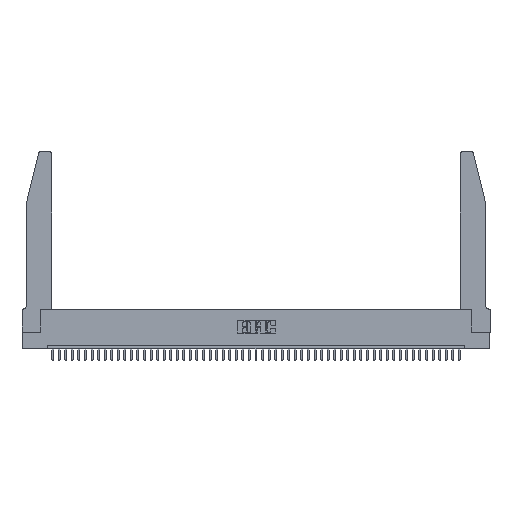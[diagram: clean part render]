
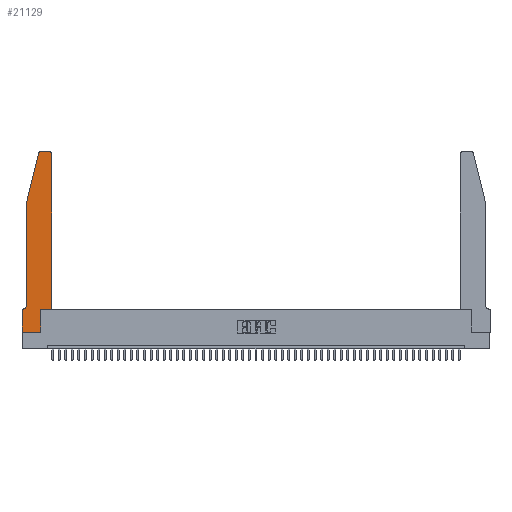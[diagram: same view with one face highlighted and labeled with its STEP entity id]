
A CAD part, top view. The second image highlights one B-rep face of the part: STEP entity #21129.
In plain terms, the highlighted planar face has unit normal (0, 0, 1).
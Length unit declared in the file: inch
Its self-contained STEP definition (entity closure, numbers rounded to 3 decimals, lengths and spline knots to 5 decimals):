
#786 = ORIENTED_EDGE ( 'NONE', *, *, #8176, .T. ) ;
#2566 = DIRECTION ( 'NONE',  ( 1., 0., 0. ) ) ;
#2634 = EDGE_CURVE ( 'NONE', #43806, #20962, #25922, .T. ) ;
#2810 = DIRECTION ( 'NONE',  ( 0., -1., 0. ) ) ;
#3086 = DIRECTION ( 'NONE',  ( 1., 0., 0. ) ) ;
#3744 = VECTOR ( 'NONE', #28747, 39.37008 ) ;
#3785 = CARTESIAN_POINT ( 'NONE',  ( 0.2865, 0.35, 0.37 ) ) ;
#3794 = VERTEX_POINT ( 'NONE', #37630 ) ;
#4685 = EDGE_CURVE ( 'NONE', #48485, #11136, #18845, .T. ) ;
#4690 = EDGE_CURVE ( 'NONE', #10500, #24135, #42140, .T. ) ;
#5651 = EDGE_CURVE ( 'NONE', #22814, #15166, #36626, .T. ) ;
#6064 = CIRCLE ( 'NONE', #27323, 0.03 ) ;
#6842 = DIRECTION ( 'NONE',  ( -1., 0., 0. ) ) ;
#6861 = CARTESIAN_POINT ( 'NONE',  ( 0.0055, 0.35, 0.37 ) ) ;
#7062 = CARTESIAN_POINT ( 'NONE',  ( 0.284, 2.72, 0.37 ) ) ;
#7360 = DIRECTION ( 'NONE',  ( 0., 1., 0. ) ) ;
#7755 = CARTESIAN_POINT ( 'NONE',  ( 0.4505, 0.35, 0.37 ) ) ;
#8176 = EDGE_CURVE ( 'NONE', #20939, #10500, #29077, .T. ) ;
#8830 = VECTOR ( 'NONE', #18913, 39.37008 ) ;
#8953 = CARTESIAN_POINT ( 'NONE',  ( 0., 0.35, 0.37 ) ) ;
#9318 = ORIENTED_EDGE ( 'NONE', *, *, #38672, .T. ) ;
#9411 = ORIENTED_EDGE ( 'NONE', *, *, #49438, .T. ) ;
#10112 = VECTOR ( 'NONE', #2810, 39.37008 ) ;
#10374 = AXIS2_PLACEMENT_3D ( 'NONE', #46440, #11872, #15708 ) ;
#10500 = VERTEX_POINT ( 'NONE', #46540 ) ;
#10507 = VECTOR ( 'NONE', #21748, 39.37008 ) ;
#10679 = CARTESIAN_POINT ( 'NONE',  ( 0., 0.35, 0.37 ) ) ;
#11030 = CIRCLE ( 'NONE', #30099, 0.03 ) ;
#11136 = VERTEX_POINT ( 'NONE', #22703 ) ;
#11353 = ORIENTED_EDGE ( 'NONE', *, *, #36166, .T. ) ;
#11358 = LINE ( 'NONE', #40221, #37043 ) ;
#11459 = DIRECTION ( 'NONE',  ( -1., 0., 0. ) ) ;
#11872 = DIRECTION ( 'NONE',  ( 0., 0., -1. ) ) ;
#12272 = CARTESIAN_POINT ( 'NONE',  ( 0.0755, 2., 0.37 ) ) ;
#12304 = LINE ( 'NONE', #49321, #35554 ) ;
#13378 = EDGE_CURVE ( 'NONE', #24135, #41936, #22000, .T. ) ;
#13555 = ORIENTED_EDGE ( 'NONE', *, *, #2634, .T. ) ;
#13577 = VECTOR ( 'NONE', #11459, 39.37008 ) ;
#14092 = EDGE_CURVE ( 'NONE', #11136, #22814, #12304, .T. ) ;
#14748 = CARTESIAN_POINT ( 'NONE',  ( 0.4505, 0.35, 0.37 ) ) ;
#15166 = VERTEX_POINT ( 'NONE', #7755 ) ;
#15403 = EDGE_LOOP ( 'NONE', ( #13555, #43340, #9318, #786, #43519, #43462, #38502, #45732, #43210, #43714, #9411, #11353 ) ) ;
#15708 = DIRECTION ( 'NONE',  ( -1., 0., 0. ) ) ;
#15936 = CARTESIAN_POINT ( 'NONE',  ( 0., 0., 0.37 ) ) ;
#17171 = DIRECTION ( 'NONE',  ( -0.239, -0.971, 0. ) ) ;
#17868 = VECTOR ( 'NONE', #6842, 39.37008 ) ;
#18358 = DIRECTION ( 'NONE',  ( 0., 0., 1. ) ) ;
#18657 = FACE_OUTER_BOUND ( 'NONE', #15403, .T. ) ;
#18824 = DIRECTION ( 'NONE',  ( 0., 0., 1. ) ) ;
#18845 = LINE ( 'NONE', #45037, #27773 ) ;
#18913 = DIRECTION ( 'NONE',  ( 0., 1., 0. ) ) ;
#19234 = DIRECTION ( 'NONE',  ( 1., 0., 0. ) ) ;
#19627 = LINE ( 'NONE', #34392, #10112 ) ;
#20939 = VERTEX_POINT ( 'NONE', #12272 ) ;
#20962 = VERTEX_POINT ( 'NONE', #44047 ) ;
#21129 = ADVANCED_FACE ( 'NONE', ( #18657 ), #37215, .T. ) ;
#21478 = LINE ( 'NONE', #14748, #8830 ) ;
#21748 = DIRECTION ( 'NONE',  ( 0., -1., 0. ) ) ;
#22000 = LINE ( 'NONE', #23900, #13577 ) ;
#22389 = DIRECTION ( 'NONE',  ( 1., 0., 0. ) ) ;
#22419 = EDGE_CURVE ( 'NONE', #41936, #48485, #19627, .T. ) ;
#22703 = CARTESIAN_POINT ( 'NONE',  ( 0.2865, 0., 0.37 ) ) ;
#22814 = VERTEX_POINT ( 'NONE', #3785 ) ;
#23683 = CARTESIAN_POINT ( 'NONE',  ( 0.4205, 2.72, 0.37 ) ) ;
#23900 = CARTESIAN_POINT ( 'NONE',  ( 0.0755, 0.35, 0.37 ) ) ;
#24135 = VERTEX_POINT ( 'NONE', #6861 ) ;
#24213 = CARTESIAN_POINT ( 'NONE',  ( 0.0755, 2., 0.37 ) ) ;
#25922 = LINE ( 'NONE', #33301, #17868 ) ;
#27323 = AXIS2_PLACEMENT_3D ( 'NONE', #7062, #18824, #3086 ) ;
#27773 = VECTOR ( 'NONE', #2566, 39.37008 ) ;
#28747 = DIRECTION ( 'NONE',  ( 1., 0., 0. ) ) ;
#29077 = LINE ( 'NONE', #24213, #10507 ) ;
#29097 = CARTESIAN_POINT ( 'NONE',  ( 0.4205, 2.75, 0.37 ) ) ;
#30099 = AXIS2_PLACEMENT_3D ( 'NONE', #23683, #46403, #19234 ) ;
#30186 = CARTESIAN_POINT ( 'NONE',  ( 0.4505, 2.72, 0.37 ) ) ;
#33301 = CARTESIAN_POINT ( 'NONE',  ( 0.2605, 2.75, 0.37 ) ) ;
#34392 = CARTESIAN_POINT ( 'NONE',  ( 0., 0., 0.37 ) ) ;
#35554 = VECTOR ( 'NONE', #7360, 39.37008 ) ;
#36166 = EDGE_CURVE ( 'NONE', #48761, #43806, #11030, .T. ) ;
#36626 = LINE ( 'NONE', #41989, #3744 ) ;
#37043 = VECTOR ( 'NONE', #17171, 39.37008 ) ;
#37215 = PLANE ( 'NONE',  #43567 ) ;
#37630 = CARTESIAN_POINT ( 'NONE',  ( 0.25487, 2.72718, 0.37 ) ) ;
#38502 = ORIENTED_EDGE ( 'NONE', *, *, #22419, .T. ) ;
#38672 = EDGE_CURVE ( 'NONE', #3794, #20939, #11358, .T. ) ;
#40221 = CARTESIAN_POINT ( 'NONE',  ( 0.0755, 2., 0.37 ) ) ;
#41936 = VERTEX_POINT ( 'NONE', #8953 ) ;
#41989 = CARTESIAN_POINT ( 'NONE',  ( 0.4505, 0.35, 0.37 ) ) ;
#42140 = CIRCLE ( 'NONE', #10374, 0.07 ) ;
#42773 = EDGE_CURVE ( 'NONE', #20962, #3794, #6064, .T. ) ;
#43210 = ORIENTED_EDGE ( 'NONE', *, *, #14092, .T. ) ;
#43340 = ORIENTED_EDGE ( 'NONE', *, *, #42773, .T. ) ;
#43462 = ORIENTED_EDGE ( 'NONE', *, *, #13378, .T. ) ;
#43519 = ORIENTED_EDGE ( 'NONE', *, *, #4690, .T. ) ;
#43567 = AXIS2_PLACEMENT_3D ( 'NONE', #10679, #18358, #22389 ) ;
#43714 = ORIENTED_EDGE ( 'NONE', *, *, #5651, .T. ) ;
#43806 = VERTEX_POINT ( 'NONE', #29097 ) ;
#44047 = CARTESIAN_POINT ( 'NONE',  ( 0.284, 2.75, 0.37 ) ) ;
#45037 = CARTESIAN_POINT ( 'NONE',  ( 0., 0., 0.37 ) ) ;
#45732 = ORIENTED_EDGE ( 'NONE', *, *, #4685, .T. ) ;
#46403 = DIRECTION ( 'NONE',  ( 0., 0., 1. ) ) ;
#46440 = CARTESIAN_POINT ( 'NONE',  ( 0.0055, 0.42, 0.37 ) ) ;
#46540 = CARTESIAN_POINT ( 'NONE',  ( 0.0755, 0.42, 0.37 ) ) ;
#48485 = VERTEX_POINT ( 'NONE', #15936 ) ;
#48761 = VERTEX_POINT ( 'NONE', #30186 ) ;
#49321 = CARTESIAN_POINT ( 'NONE',  ( 0.2865, 0.35, 0.37 ) ) ;
#49438 = EDGE_CURVE ( 'NONE', #15166, #48761, #21478, .T. ) ;
